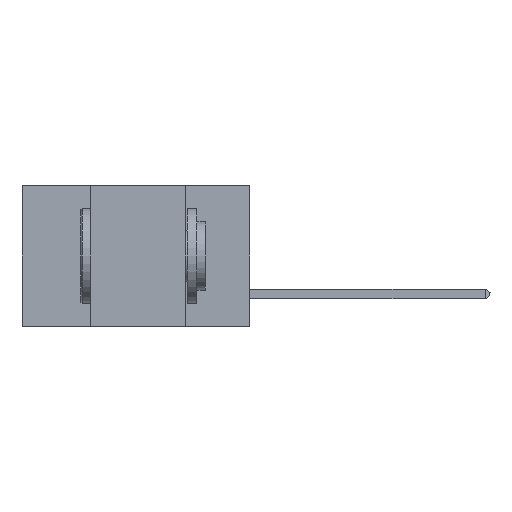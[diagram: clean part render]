
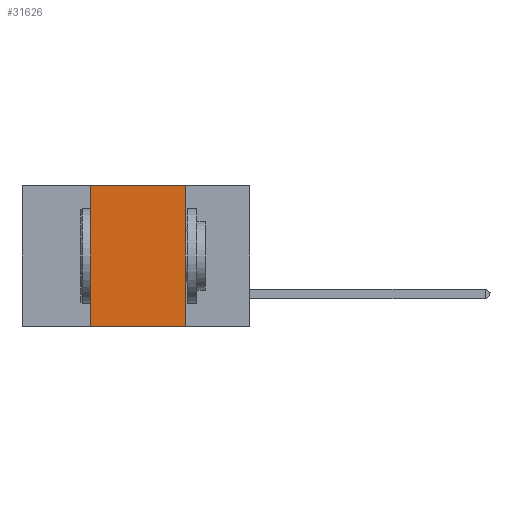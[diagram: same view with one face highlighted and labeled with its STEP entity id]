
A CAD part, left-side view. The second image highlights one B-rep face of the part: STEP entity #31626.
In plain terms, the highlighted planar face has unit normal (-1, 0, 0).
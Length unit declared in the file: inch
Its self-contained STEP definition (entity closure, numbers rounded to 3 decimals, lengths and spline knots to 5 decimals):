
#1635 = DIRECTION ( 'NONE',  ( 0., 0., -1. ) ) ;
#1794 = DIRECTION ( 'NONE',  ( 1., 0., 0. ) ) ;
#2405 = EDGE_CURVE ( 'NONE', #32682, #2704, #6420, .T. ) ;
#2704 = VERTEX_POINT ( 'NONE', #3836 ) ;
#3190 = VERTEX_POINT ( 'NONE', #18794 ) ;
#3836 = CARTESIAN_POINT ( 'NONE',  ( 0., 0.42, 0. ) ) ;
#4356 = VECTOR ( 'NONE', #34415, 39.37008 ) ;
#6420 = LINE ( 'NONE', #32256, #34046 ) ;
#6733 = EDGE_CURVE ( 'NONE', #2704, #7237, #11046, .T. ) ;
#7237 = VERTEX_POINT ( 'NONE', #11692 ) ;
#7915 = CARTESIAN_POINT ( 'NONE',  ( 0., 0.17, 0. ) ) ;
#8025 = CARTESIAN_POINT ( 'NONE',  ( 0., 0.6, -0.37 ) ) ;
#11046 = LINE ( 'NONE', #19526, #4356 ) ;
#11190 = EDGE_CURVE ( 'NONE', #7237, #3190, #41720, .T. ) ;
#11692 = CARTESIAN_POINT ( 'NONE',  ( 0., 0.17, 0. ) ) ;
#13308 = VECTOR ( 'NONE', #36737, 39.37008 ) ;
#18794 = CARTESIAN_POINT ( 'NONE',  ( 0., 0.17, -0.37 ) ) ;
#19526 = CARTESIAN_POINT ( 'NONE',  ( 0., 0.6, 0. ) ) ;
#21377 = CARTESIAN_POINT ( 'NONE',  ( 0., 0.42, -0.37 ) ) ;
#23131 = PLANE ( 'NONE',  #37608 ) ;
#23543 = EDGE_LOOP ( 'NONE', ( #31615, #44111, #35478, #32638 ) ) ;
#29117 = DIRECTION ( 'NONE',  ( 0., 0., 1. ) ) ;
#30817 = FACE_OUTER_BOUND ( 'NONE', #23543, .T. ) ;
#31547 = VECTOR ( 'NONE', #43691, 39.37008 ) ;
#31615 = ORIENTED_EDGE ( 'NONE', *, *, #11190, .F. ) ;
#31626 = ADVANCED_FACE ( 'NONE', ( #30817 ), #23131, .F. ) ;
#32139 = EDGE_CURVE ( 'NONE', #32682, #3190, #39225, .T. ) ;
#32256 = CARTESIAN_POINT ( 'NONE',  ( 0., 0.42, 0. ) ) ;
#32638 = ORIENTED_EDGE ( 'NONE', *, *, #32139, .T. ) ;
#32682 = VERTEX_POINT ( 'NONE', #21377 ) ;
#33769 = CARTESIAN_POINT ( 'NONE',  ( 0., 0.6, 0. ) ) ;
#34046 = VECTOR ( 'NONE', #29117, 39.37008 ) ;
#34415 = DIRECTION ( 'NONE',  ( 0., -1., 0. ) ) ;
#35478 = ORIENTED_EDGE ( 'NONE', *, *, #2405, .F. ) ;
#36737 = DIRECTION ( 'NONE',  ( 0., -1., 0. ) ) ;
#37608 = AXIS2_PLACEMENT_3D ( 'NONE', #33769, #1794, #1635 ) ;
#39225 = LINE ( 'NONE', #8025, #13308 ) ;
#41720 = LINE ( 'NONE', #7915, #31547 ) ;
#43691 = DIRECTION ( 'NONE',  ( 0., 0., -1. ) ) ;
#44111 = ORIENTED_EDGE ( 'NONE', *, *, #6733, .F. ) ;
